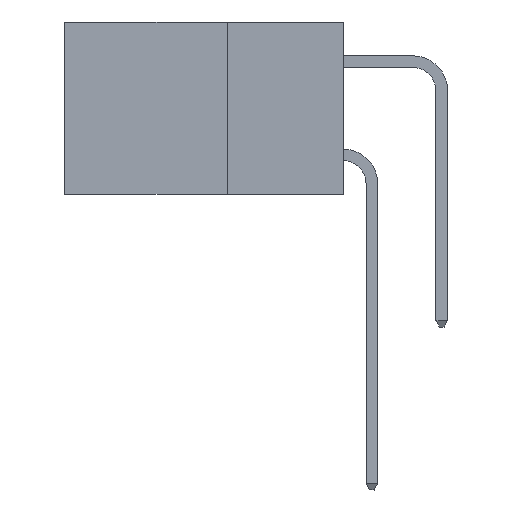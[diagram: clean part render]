
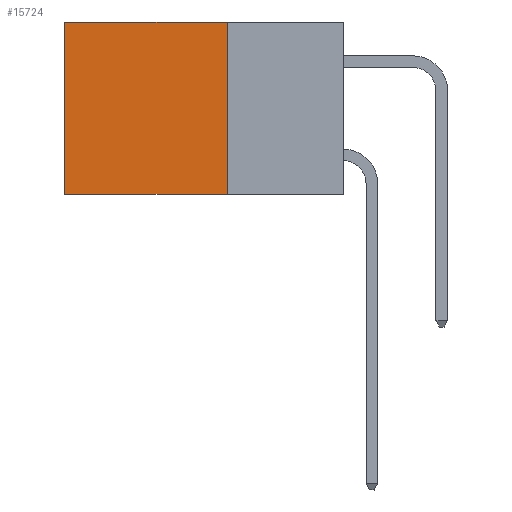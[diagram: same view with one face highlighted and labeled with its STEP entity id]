
A CAD part, left-side view. The second image highlights one B-rep face of the part: STEP entity #15724.
In plain terms, the highlighted planar face has unit normal (-1, 0, 0).
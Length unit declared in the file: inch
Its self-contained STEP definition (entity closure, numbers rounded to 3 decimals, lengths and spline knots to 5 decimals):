
#815 = LINE ( 'NONE', #3841, #8862 ) ;
#1582 = ORIENTED_EDGE ( 'NONE', *, *, #4953, .T. ) ;
#2566 = CARTESIAN_POINT ( 'NONE',  ( 0.298, 0.6, 0. ) ) ;
#3841 = CARTESIAN_POINT ( 'NONE',  ( 0.298, 0.6, 0. ) ) ;
#3846 = VECTOR ( 'NONE', #3882, 39.37008 ) ;
#3882 = DIRECTION ( 'NONE',  ( 0., 0., -1. ) ) ;
#4953 = EDGE_CURVE ( 'NONE', #6330, #10314, #27951, .T. ) ;
#6330 = VERTEX_POINT ( 'NONE', #29559 ) ;
#6779 = PLANE ( 'NONE',  #9807 ) ;
#8862 = VECTOR ( 'NONE', #18309, 39.37008 ) ;
#9034 = CARTESIAN_POINT ( 'NONE',  ( 0.298, 0.6, -0.37 ) ) ;
#9362 = FACE_OUTER_BOUND ( 'NONE', #26729, .T. ) ;
#9807 = AXIS2_PLACEMENT_3D ( 'NONE', #28191, #25965, #11696 ) ;
#10314 = VERTEX_POINT ( 'NONE', #2566 ) ;
#10803 = ORIENTED_EDGE ( 'NONE', *, *, #18553, .F. ) ;
#11230 = CARTESIAN_POINT ( 'NONE',  ( 0.298, 0.25, 0. ) ) ;
#11696 = DIRECTION ( 'NONE',  ( 0., 0., -1. ) ) ;
#11746 = CARTESIAN_POINT ( 'NONE',  ( 0.298, 0.25, 0. ) ) ;
#12299 = EDGE_CURVE ( 'NONE', #17490, #28545, #20977, .T. ) ;
#14666 = VECTOR ( 'NONE', #28990, 39.37008 ) ;
#15382 = VECTOR ( 'NONE', #28350, 39.37008 ) ;
#15724 = ADVANCED_FACE ( 'NONE', ( #9362 ), #6779, .F. ) ;
#17287 = EDGE_CURVE ( 'NONE', #10314, #28545, #815, .T. ) ;
#17490 = VERTEX_POINT ( 'NONE', #23738 ) ;
#18309 = DIRECTION ( 'NONE',  ( 0., 0., -1. ) ) ;
#18553 = EDGE_CURVE ( 'NONE', #6330, #17490, #22333, .T. ) ;
#20977 = LINE ( 'NONE', #24304, #14666 ) ;
#22333 = LINE ( 'NONE', #11230, #3846 ) ;
#23738 = CARTESIAN_POINT ( 'NONE',  ( 0.298, 0.25, -0.37 ) ) ;
#23746 = ORIENTED_EDGE ( 'NONE', *, *, #17287, .T. ) ;
#24304 = CARTESIAN_POINT ( 'NONE',  ( 0.298, 0.25, -0.37 ) ) ;
#25965 = DIRECTION ( 'NONE',  ( 1., 0., 0. ) ) ;
#26729 = EDGE_LOOP ( 'NONE', ( #23746, #27512, #10803, #1582 ) ) ;
#27512 = ORIENTED_EDGE ( 'NONE', *, *, #12299, .F. ) ;
#27951 = LINE ( 'NONE', #11746, #15382 ) ;
#28191 = CARTESIAN_POINT ( 'NONE',  ( 0.298, 0.25, 0. ) ) ;
#28350 = DIRECTION ( 'NONE',  ( 0., 1., 0. ) ) ;
#28545 = VERTEX_POINT ( 'NONE', #9034 ) ;
#28990 = DIRECTION ( 'NONE',  ( 0., 1., 0. ) ) ;
#29559 = CARTESIAN_POINT ( 'NONE',  ( 0.298, 0.25, 0. ) ) ;
